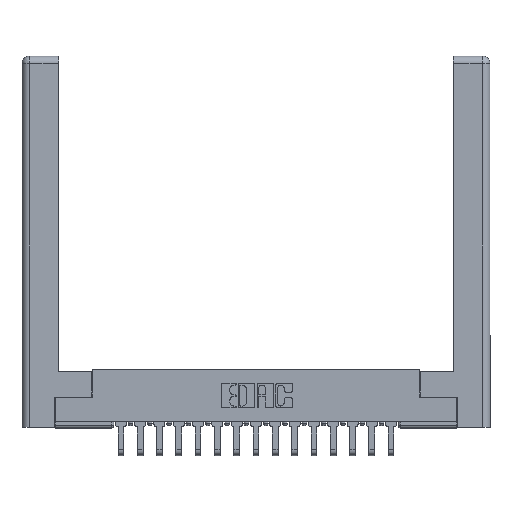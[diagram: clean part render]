
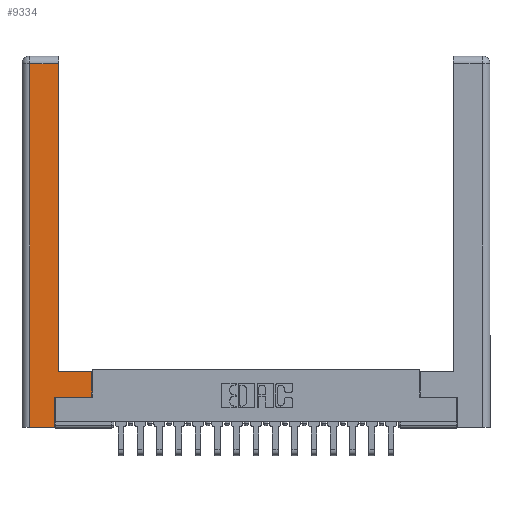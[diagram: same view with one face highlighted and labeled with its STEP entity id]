
A CAD part, top view. The second image highlights one B-rep face of the part: STEP entity #9334.
In plain terms, the highlighted planar face has unit normal (0, 0, 1).
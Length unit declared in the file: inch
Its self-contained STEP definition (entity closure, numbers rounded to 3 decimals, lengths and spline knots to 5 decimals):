
#8 = CARTESIAN_POINT ( 'NONE',  ( 0.565, 0.245, 0. ) ) ;
#64 = VECTOR ( 'NONE', #8642, 39.37008 ) ;
#68 = LINE ( 'NONE', #6488, #20610 ) ;
#280 = DIRECTION ( 'NONE',  ( 0., -1., 0. ) ) ;
#470 = VERTEX_POINT ( 'NONE', #4981 ) ;
#789 = DIRECTION ( 'NONE',  ( 0., 1., 0. ) ) ;
#1280 = LINE ( 'NONE', #9166, #6784 ) ;
#1358 = AXIS2_PLACEMENT_3D ( 'NONE', #19760, #17637, #3242 ) ;
#1534 = CARTESIAN_POINT ( 'NONE',  ( 0.565, 0.45, 0. ) ) ;
#1985 = DIRECTION ( 'NONE',  ( -1., 0., 0. ) ) ;
#2061 = DIRECTION ( 'NONE',  ( -1., 0., 0. ) ) ;
#2151 = VERTEX_POINT ( 'NONE', #8 ) ;
#2170 = VECTOR ( 'NONE', #18370, 39.37008 ) ;
#2668 = CARTESIAN_POINT ( 'NONE',  ( 0.265, 0., 0. ) ) ;
#3242 = DIRECTION ( 'NONE',  ( -1., 0., 0. ) ) ;
#3251 = VERTEX_POINT ( 'NONE', #4466 ) ;
#3395 = VERTEX_POINT ( 'NONE', #5268 ) ;
#3956 = LINE ( 'NONE', #11831, #11690 ) ;
#4080 = LINE ( 'NONE', #17008, #2170 ) ;
#4278 = ORIENTED_EDGE ( 'NONE', *, *, #16985, .T. ) ;
#4466 = CARTESIAN_POINT ( 'NONE',  ( 0.0615, 0., 0. ) ) ;
#4823 = ORIENTED_EDGE ( 'NONE', *, *, #11303, .T. ) ;
#4981 = CARTESIAN_POINT ( 'NONE',  ( 0.265, 0.245, 0. ) ) ;
#5098 = LINE ( 'NONE', #13083, #11081 ) ;
#5250 = VERTEX_POINT ( 'NONE', #13764 ) ;
#5268 = CARTESIAN_POINT ( 'NONE',  ( 0.295, 0.45, 0. ) ) ;
#5384 = ORIENTED_EDGE ( 'NONE', *, *, #12685, .T. ) ;
#6182 = FACE_OUTER_BOUND ( 'NONE', #15362, .T. ) ;
#6488 = CARTESIAN_POINT ( 'NONE',  ( 0.295, 3., 0. ) ) ;
#6652 = CARTESIAN_POINT ( 'NONE',  ( 0.295, 2.94, 0. ) ) ;
#6771 = VECTOR ( 'NONE', #1985, 39.37008 ) ;
#6780 = ORIENTED_EDGE ( 'NONE', *, *, #13159, .T. ) ;
#6784 = VECTOR ( 'NONE', #13893, 39.37008 ) ;
#7457 = EDGE_CURVE ( 'NONE', #2151, #9854, #3956, .T. ) ;
#7799 = CARTESIAN_POINT ( 'NONE',  ( 0.0615, 2.94, 0. ) ) ;
#8147 = ORIENTED_EDGE ( 'NONE', *, *, #7457, .T. ) ;
#8232 = VERTEX_POINT ( 'NONE', #7799 ) ;
#8385 = VECTOR ( 'NONE', #280, 39.37008 ) ;
#8642 = DIRECTION ( 'NONE',  ( 1., 0., 0. ) ) ;
#9080 = ORIENTED_EDGE ( 'NONE', *, *, #9428, .T. ) ;
#9166 = CARTESIAN_POINT ( 'NONE',  ( 0.565, 0.245, 0. ) ) ;
#9334 = ADVANCED_FACE ( 'NONE', ( #6182 ), #12589, .F. ) ;
#9428 = EDGE_CURVE ( 'NONE', #8232, #3251, #14789, .T. ) ;
#9854 = VERTEX_POINT ( 'NONE', #1534 ) ;
#9963 = LINE ( 'NONE', #16379, #6771 ) ;
#11081 = VECTOR ( 'NONE', #2061, 39.37008 ) ;
#11303 = EDGE_CURVE ( 'NONE', #19244, #8232, #5098, .T. ) ;
#11690 = VECTOR ( 'NONE', #789, 39.37008 ) ;
#11831 = CARTESIAN_POINT ( 'NONE',  ( 0.565, 0.45, 0. ) ) ;
#12589 = PLANE ( 'NONE',  #1358 ) ;
#12685 = EDGE_CURVE ( 'NONE', #9854, #3395, #9963, .T. ) ;
#13083 = CARTESIAN_POINT ( 'NONE',  ( 0.0615, 2.94, 0. ) ) ;
#13159 = EDGE_CURVE ( 'NONE', #3251, #5250, #18329, .T. ) ;
#13317 = DIRECTION ( 'NONE',  ( 0., 1., 0. ) ) ;
#13383 = EDGE_CURVE ( 'NONE', #470, #2151, #1280, .T. ) ;
#13764 = CARTESIAN_POINT ( 'NONE',  ( 0.265, 0., 0. ) ) ;
#13893 = DIRECTION ( 'NONE',  ( 1., 0., 0. ) ) ;
#14081 = ORIENTED_EDGE ( 'NONE', *, *, #13383, .T. ) ;
#14789 = LINE ( 'NONE', #16367, #8385 ) ;
#15362 = EDGE_LOOP ( 'NONE', ( #4278, #4823, #9080, #6780, #17605, #14081, #8147, #5384 ) ) ;
#16367 = CARTESIAN_POINT ( 'NONE',  ( 0.0615, 0., 0. ) ) ;
#16379 = CARTESIAN_POINT ( 'NONE',  ( 0.295, 0.45, 0. ) ) ;
#16985 = EDGE_CURVE ( 'NONE', #3395, #19244, #68, .T. ) ;
#17008 = CARTESIAN_POINT ( 'NONE',  ( 0.265, 0.245, 0. ) ) ;
#17159 = EDGE_CURVE ( 'NONE', #5250, #470, #4080, .T. ) ;
#17605 = ORIENTED_EDGE ( 'NONE', *, *, #17159, .T. ) ;
#17637 = DIRECTION ( 'NONE',  ( 0., 0., -1. ) ) ;
#18329 = LINE ( 'NONE', #2668, #64 ) ;
#18370 = DIRECTION ( 'NONE',  ( 0., 1., 0. ) ) ;
#19244 = VERTEX_POINT ( 'NONE', #6652 ) ;
#19760 = CARTESIAN_POINT ( 'NONE',  ( 0., 0., 0. ) ) ;
#20610 = VECTOR ( 'NONE', #13317, 39.37008 ) ;
